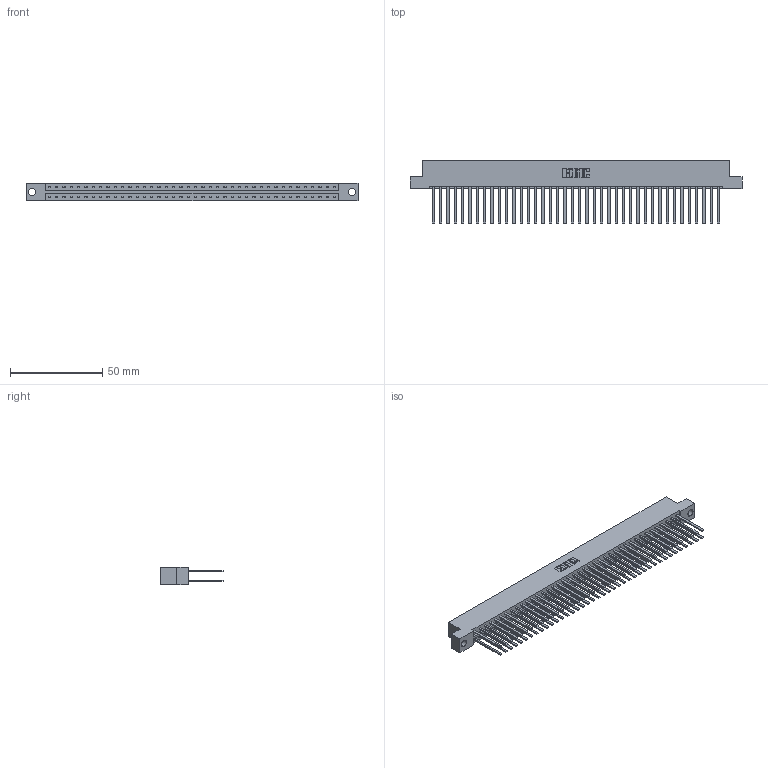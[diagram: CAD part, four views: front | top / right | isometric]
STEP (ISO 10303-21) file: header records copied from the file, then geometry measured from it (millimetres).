
FILE_DESCRIPTION (( 'STEP AP203' ), '1' );
FILE_NAME ('333-080-544-204.STEP', '2018-08-05T01:51:37', ( '' ), ( '' ), 'SwSTEP 2.0', 'SolidWorks 2016', '' );
FILE_SCHEMA (( 'CONFIG_CONTROL_DESIGN' ));
Length unit declared in the file: inch
Products named in the file (3): 333-080-544-204; 333 Part_Flush - .156 Dia - TH; 345-292-001_345-293-144
Assembly tree (81 placements, depth 2):
  333-080-544-204
    333 Part_Flush - .156 Dia - TH
    345-292-001_345-293-144  x80
Bounding box: 180.04 x 34.3 x 9.4 mm (x, y, z)
Volume: 19395.5 mm3; surface area: 26319 mm2
Topology: 81 solids, 81 shells, 3794 faces, 11271 edges, 7406 vertices
Faces by surface type: plane 2630, cylinder 1164
Entity records: 25811 total; most frequent: CARTESIAN_POINT 4278, ORIENTED_EDGE 4214, DIRECTION 3655, EDGE_CURVE 2107, LINE 1983, VECTOR 1983, VERTEX_POINT 1402, AXIS2_PLACEMENT_3D 836
